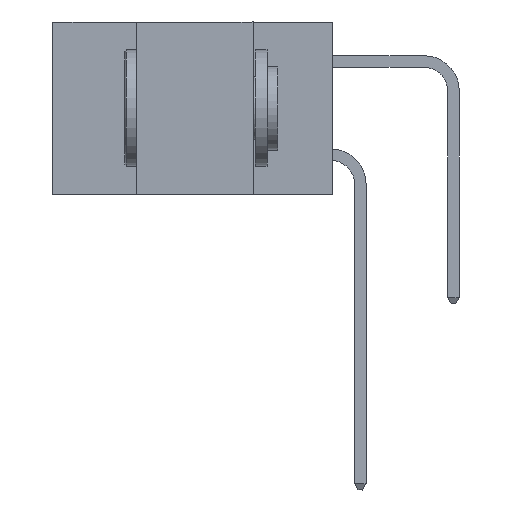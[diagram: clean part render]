
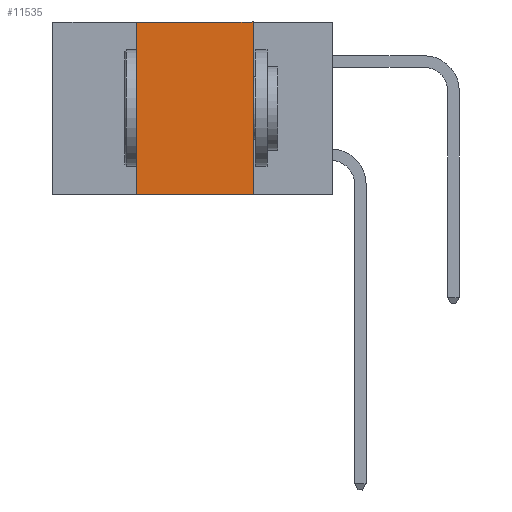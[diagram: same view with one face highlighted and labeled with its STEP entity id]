
A CAD part, left-side view. The second image highlights one B-rep face of the part: STEP entity #11535.
In plain terms, the highlighted planar face has unit normal (-1, 0, 0).
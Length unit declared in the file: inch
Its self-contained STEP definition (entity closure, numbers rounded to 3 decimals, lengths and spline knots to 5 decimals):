
#237 = CARTESIAN_POINT ( 'NONE',  ( 0., 0.6, 0. ) ) ;
#456 = LINE ( 'NONE', #4690, #10709 ) ;
#691 = ORIENTED_EDGE ( 'NONE', *, *, #821, .F. ) ;
#821 = EDGE_CURVE ( 'NONE', #7637, #3200, #456, .T. ) ;
#1559 = PLANE ( 'NONE',  #2372 ) ;
#2372 = AXIS2_PLACEMENT_3D ( 'NONE', #237, #3628, #2520 ) ;
#2520 = DIRECTION ( 'NONE',  ( 0., 0., -1. ) ) ;
#2733 = DIRECTION ( 'NONE',  ( 0., -1., 0. ) ) ;
#3200 = VERTEX_POINT ( 'NONE', #12439 ) ;
#3588 = CARTESIAN_POINT ( 'NONE',  ( 0., 0.17, -0.37 ) ) ;
#3628 = DIRECTION ( 'NONE',  ( 1., 0., 0. ) ) ;
#4540 = FACE_OUTER_BOUND ( 'NONE', #7245, .T. ) ;
#4690 = CARTESIAN_POINT ( 'NONE',  ( 0., 0.42, -0.37 ) ) ;
#4993 = LINE ( 'NONE', #9028, #11004 ) ;
#5313 = ORIENTED_EDGE ( 'NONE', *, *, #12127, .F. ) ;
#5914 = CARTESIAN_POINT ( 'NONE',  ( 0., 0.6, -0.37 ) ) ;
#6918 = VERTEX_POINT ( 'NONE', #3588 ) ;
#7245 = EDGE_LOOP ( 'NONE', ( #7902, #5313, #691, #11473 ) ) ;
#7467 = EDGE_CURVE ( 'NONE', #7637, #6918, #9054, .T. ) ;
#7637 = VERTEX_POINT ( 'NONE', #9472 ) ;
#7902 = ORIENTED_EDGE ( 'NONE', *, *, #13646, .F. ) ;
#9028 = CARTESIAN_POINT ( 'NONE',  ( 0., 0.6, 0. ) ) ;
#9054 = LINE ( 'NONE', #5914, #10831 ) ;
#9472 = CARTESIAN_POINT ( 'NONE',  ( 0., 0.42, -0.37 ) ) ;
#9984 = CARTESIAN_POINT ( 'NONE',  ( 0., 0.17, 0. ) ) ;
#10154 = VECTOR ( 'NONE', #11394, 39.37008 ) ;
#10189 = DIRECTION ( 'NONE',  ( 0., -1., 0. ) ) ;
#10709 = VECTOR ( 'NONE', #13365, 39.37008 ) ;
#10726 = VERTEX_POINT ( 'NONE', #9984 ) ;
#10831 = VECTOR ( 'NONE', #2733, 39.37008 ) ;
#11004 = VECTOR ( 'NONE', #10189, 39.37008 ) ;
#11394 = DIRECTION ( 'NONE',  ( 0., 0., -1. ) ) ;
#11470 = LINE ( 'NONE', #12290, #10154 ) ;
#11473 = ORIENTED_EDGE ( 'NONE', *, *, #7467, .T. ) ;
#11535 = ADVANCED_FACE ( 'NONE', ( #4540 ), #1559, .F. ) ;
#12127 = EDGE_CURVE ( 'NONE', #3200, #10726, #4993, .T. ) ;
#12290 = CARTESIAN_POINT ( 'NONE',  ( 0., 0.17, -0.37 ) ) ;
#12439 = CARTESIAN_POINT ( 'NONE',  ( 0., 0.42, 0. ) ) ;
#13365 = DIRECTION ( 'NONE',  ( 0., 0., 1. ) ) ;
#13646 = EDGE_CURVE ( 'NONE', #10726, #6918, #11470, .T. ) ;
